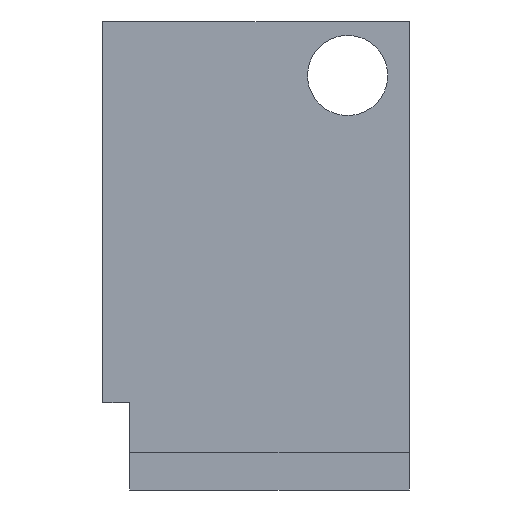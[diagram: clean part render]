
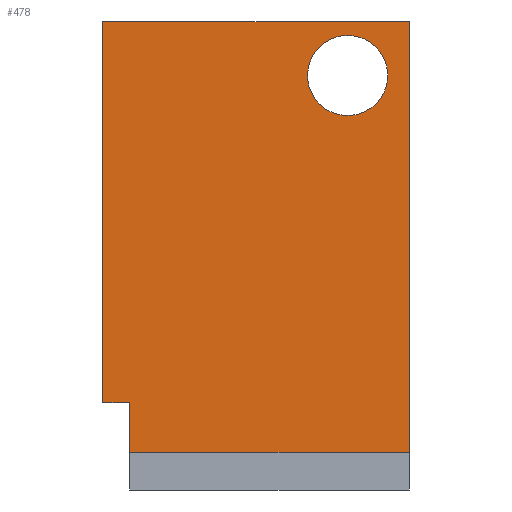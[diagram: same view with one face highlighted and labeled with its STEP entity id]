
A CAD part, front view. The second image highlights one B-rep face of the part: STEP entity #478.
In plain terms, the highlighted planar face has unit normal (0, -1, 0).
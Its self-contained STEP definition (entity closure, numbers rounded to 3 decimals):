
#15=FACE_BOUND('',#69,.T.);
#21=CIRCLE('',#521,1.5);
#44=FACE_OUTER_BOUND('',#68,.T.);
#68=EDGE_LOOP('',(#390,#391,#392,#393,#394,#395));
#69=EDGE_LOOP('',(#396));
#93=LINE('',#715,#149);
#101=LINE('',#731,#157);
#109=LINE('',#749,#165);
#113=LINE('',#757,#169);
#123=LINE('',#779,#179);
#127=LINE('',#787,#183);
#149=VECTOR('',#567,10.);
#157=VECTOR('',#579,10.);
#165=VECTOR('',#597,10.);
#169=VECTOR('',#605,10.);
#179=VECTOR('',#625,10.);
#183=VECTOR('',#637,10.);
#206=VERTEX_POINT('',#712);
#207=VERTEX_POINT('',#714);
#212=VERTEX_POINT('',#728);
#213=VERTEX_POINT('',#730);
#218=VERTEX_POINT('',#748);
#220=VERTEX_POINT('',#756);
#226=VERTEX_POINT('',#772);
#251=EDGE_CURVE('',#207,#206,#93,.T.);
#259=EDGE_CURVE('',#213,#212,#101,.T.);
#268=EDGE_CURVE('',#212,#218,#109,.T.);
#272=EDGE_CURVE('',#218,#220,#113,.T.);
#280=EDGE_CURVE('',#226,#226,#21,.T.);
#284=EDGE_CURVE('',#220,#207,#123,.T.);
#288=EDGE_CURVE('',#206,#213,#127,.T.);
#390=ORIENTED_EDGE('',*,*,#272,.T.);
#391=ORIENTED_EDGE('',*,*,#284,.T.);
#392=ORIENTED_EDGE('',*,*,#251,.T.);
#393=ORIENTED_EDGE('',*,*,#288,.T.);
#394=ORIENTED_EDGE('',*,*,#259,.T.);
#395=ORIENTED_EDGE('',*,*,#268,.T.);
#396=ORIENTED_EDGE('',*,*,#280,.T.);
#432=PLANE('',#527);
#478=ADVANCED_FACE('',(#44,#15),#432,.T.);
#521=AXIS2_PLACEMENT_3D('',#773,#617,#618);
#527=AXIS2_PLACEMENT_3D('',#786,#635,#636);
#567=DIRECTION('',(0.,0.,1.));
#579=DIRECTION('',(0.,0.,-1.));
#597=DIRECTION('',(1.,0.,0.));
#605=DIRECTION('',(0.,0.,-1.));
#617=DIRECTION('center_axis',(0.,1.,0.));
#618=DIRECTION('ref_axis',(0.267,0.,-0.964));
#625=DIRECTION('',(1.,0.,0.));
#635=DIRECTION('center_axis',(0.,-1.,0.));
#636=DIRECTION('ref_axis',(0.,0.,1.));
#637=DIRECTION('',(-1.,0.,0.));
#712=CARTESIAN_POINT('',(37.65,-9.786,-26.052));
#714=CARTESIAN_POINT('',(37.65,-9.786,-42.142));
#715=CARTESIAN_POINT('',(37.65,-9.786,-43.988));
#728=CARTESIAN_POINT('',(26.179,-9.786,-40.302));
#730=CARTESIAN_POINT('',(26.179,-9.786,-26.052));
#731=CARTESIAN_POINT('',(26.179,-9.786,-34.188));
#748=CARTESIAN_POINT('',(27.187,-9.786,-40.302));
#749=CARTESIAN_POINT('',(35.017,-9.786,-40.302));
#756=CARTESIAN_POINT('',(27.187,-9.786,-42.142));
#757=CARTESIAN_POINT('',(27.187,-9.786,-41.722));
#772=CARTESIAN_POINT('',(34.941,-9.786,-26.607));
#773=CARTESIAN_POINT('Origin',(35.342,-9.786,-28.052));
#779=CARTESIAN_POINT('',(43.855,-9.786,-42.142));
#786=CARTESIAN_POINT('Origin',(43.855,-9.786,-43.142));
#787=CARTESIAN_POINT('',(43.855,-9.786,-26.052));
